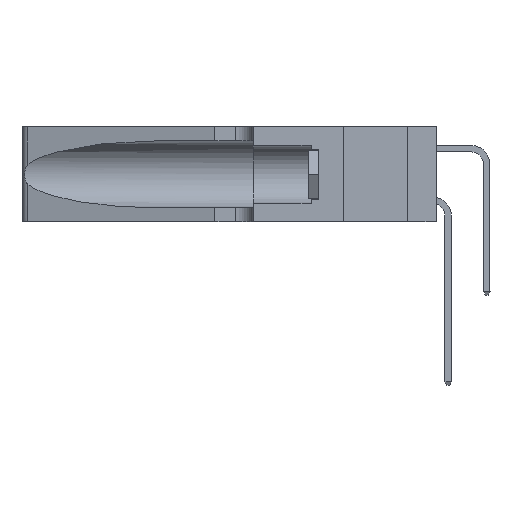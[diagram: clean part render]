
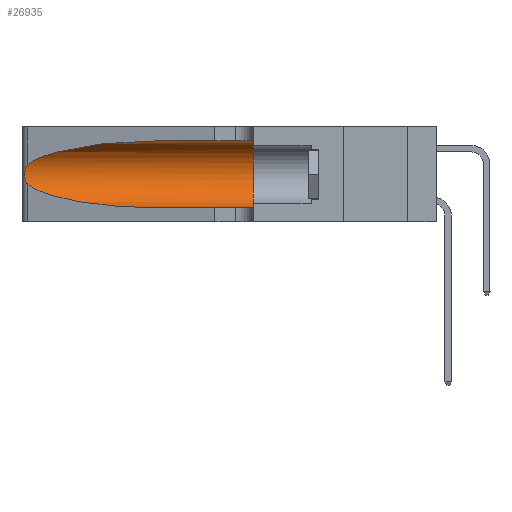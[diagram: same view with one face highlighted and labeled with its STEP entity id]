
A CAD part, left-side view. The second image highlights one B-rep face of the part: STEP entity #26935.
In plain terms, the highlighted cylindrical face has radius 3.308 mm (diameter 6.617 mm), a partial arc.
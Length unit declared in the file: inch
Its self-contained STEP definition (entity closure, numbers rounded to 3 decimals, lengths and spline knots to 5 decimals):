
#251 = ORIENTED_EDGE ( 'NONE', *, *, #4112, .T. ) ;
#1411 = CARTESIAN_POINT ( 'NONE',  ( 0.1305, 1.61858, 0.185 ) ) ;
#1829 = CARTESIAN_POINT ( 'NONE',  ( 0.25487, 1.22718, 0.14631 ) ) ;
#2220 = CARTESIAN_POINT ( 'NONE',  ( 0.25487, 1.22718, 0.14631 ) ) ;
#2361 = EDGE_CURVE ( 'NONE', #14795, #5039, #16998, .T. ) ;
#3120 = VERTEX_POINT ( 'NONE', #29177 ) ;
#3632 = CARTESIAN_POINT ( 'NONE',  ( 0.1305, 0.72297, 0.31525 ) ) ;
#4112 = EDGE_CURVE ( 'NONE', #5039, #3120, #10469, .T. ) ;
#4532 = CARTESIAN_POINT ( 'NONE',  ( 0.25639, 1.23184, 0.21858 ) ) ;
#4702 = DIRECTION ( 'NONE',  ( 0., -1., 0. ) ) ;
#5038 = EDGE_CURVE ( 'NONE', #13819, #35014, #19594, .T. ) ;
#5039 = VERTEX_POINT ( 'NONE', #11782 ) ;
#5859 = LINE ( 'NONE', #15915, #34793 ) ;
#6464 = CARTESIAN_POINT ( 'NONE',  ( 0.18966, 0.96281, 0.31525 ) ) ;
#7386 = CARTESIAN_POINT ( 'NONE',  ( 0.25854, 1.2359, 0.20912 ) ) ;
#7924 = CARTESIAN_POINT ( 'NONE',  ( 0.1305, 0.72297, 0.05475 ) ) ;
#8695 = CIRCLE ( 'NONE', #29893, 0.13025 ) ;
#9926 = DIRECTION ( 'NONE',  ( 0., 0., -1. ) ) ;
#10215 = CARTESIAN_POINT ( 'NONE',  ( 0.26075, 1.23896, 0.19203 ) ) ;
#10469 =( BOUNDED_CURVE ( )  B_SPLINE_CURVE ( 3, ( #2220, #21920, #24758, #7924 ),
 .UNSPECIFIED., .F., .F. ) 
 B_SPLINE_CURVE_WITH_KNOTS ( ( 4, 4 ),
 ( 3.44316, 4.71239 ),
 .UNSPECIFIED. ) 
 CURVE ( )  GEOMETRIC_REPRESENTATION_ITEM ( )  RATIONAL_B_SPLINE_CURVE ( ( 1., 0.87, 0.87, 1. ) ) 
 REPRESENTATION_ITEM ( '' )  );
#11574 =( BOUNDED_CURVE ( )  B_SPLINE_CURVE ( 3, ( #3632, #6464, #14979, #34494 ),
 .UNSPECIFIED., .F., .T. ) 
 B_SPLINE_CURVE_WITH_KNOTS ( ( 4, 4 ),
 ( 1.5708, 2.84003 ),
 .UNSPECIFIED. ) 
 CURVE ( )  GEOMETRIC_REPRESENTATION_ITEM ( )  RATIONAL_B_SPLINE_CURVE ( ( 1., 0.87, 0.87, 1. ) ) 
 REPRESENTATION_ITEM ( '' )  );
#11602 = DIRECTION ( 'NONE',  ( 0., 1., 0. ) ) ;
#11782 = CARTESIAN_POINT ( 'NONE',  ( 0.25487, 1.22718, 0.14631 ) ) ;
#12039 = CARTESIAN_POINT ( 'NONE',  ( 0.25487, 1.22718, 0.22369 ) ) ;
#12203 = CARTESIAN_POINT ( 'NONE',  ( 0.1305, 0.35, 0.31525 ) ) ;
#12540 = FACE_OUTER_BOUND ( 'NONE', #31478, .T. ) ;
#13046 = CARTESIAN_POINT ( 'NONE',  ( 0.26017, 1.23833, 0.17102 ) ) ;
#13693 = CARTESIAN_POINT ( 'NONE',  ( 0.1305, 0.72297, 0.31525 ) ) ;
#13819 = VERTEX_POINT ( 'NONE', #13693 ) ;
#14145 = ORIENTED_EDGE ( 'NONE', *, *, #5038, .F. ) ;
#14795 = VERTEX_POINT ( 'NONE', #12039 ) ;
#14979 = CARTESIAN_POINT ( 'NONE',  ( 0.2373, 1.15595, 0.28018 ) ) ;
#15858 = CARTESIAN_POINT ( 'NONE',  ( 0.25789, 1.23486, 0.15765 ) ) ;
#15915 = CARTESIAN_POINT ( 'NONE',  ( 0.1305, 1.61858, 0.05475 ) ) ;
#16998 = B_SPLINE_CURVE_WITH_KNOTS ( 'NONE', 3,
 ( #35282, #21401, #4532, #24237, #7386, #27033, #10215, #29806, #13046, #32613, #15858, #35395, #18716, #1829 ),
 .UNSPECIFIED., .F., .F.,
 ( 4, 2, 2, 2, 2, 2, 4 ),
 ( 0., 0.00027, 0.00053, 0.00107, 0.0016, 0.00187, 0.00214 ),
 .UNSPECIFIED. ) ;
#18716 = CARTESIAN_POINT ( 'NONE',  ( 0.25555, 1.22993, 0.14849 ) ) ;
#19594 = LINE ( 'NONE', #28569, #33545 ) ;
#19875 = ORIENTED_EDGE ( 'NONE', *, *, #2361, .T. ) ;
#21401 = CARTESIAN_POINT ( 'NONE',  ( 0.25555, 1.22994, 0.2215 ) ) ;
#21920 = CARTESIAN_POINT ( 'NONE',  ( 0.2373, 1.15595, 0.08982 ) ) ;
#22706 = ORIENTED_EDGE ( 'NONE', *, *, #25441, .F. ) ;
#24237 = CARTESIAN_POINT ( 'NONE',  ( 0.25787, 1.23484, 0.2124 ) ) ;
#24747 = VERTEX_POINT ( 'NONE', #28201 ) ;
#24758 = CARTESIAN_POINT ( 'NONE',  ( 0.18966, 0.96281, 0.05475 ) ) ;
#24858 = CYLINDRICAL_SURFACE ( 'NONE', #27260, 0.13025 ) ;
#25441 = EDGE_CURVE ( 'NONE', #35014, #24747, #8695, .T. ) ;
#26743 = DIRECTION ( 'NONE',  ( 0., -1., 0. ) ) ;
#26814 = EDGE_CURVE ( 'NONE', #13819, #14795, #11574, .T. ) ;
#26935 = ADVANCED_FACE ( 'NONE', ( #12540 ), #24858, .F. ) ;
#27033 = CARTESIAN_POINT ( 'NONE',  ( 0.26018, 1.23835, 0.19895 ) ) ;
#27260 = AXIS2_PLACEMENT_3D ( 'NONE', #1411, #26743, #9926 ) ;
#28201 = CARTESIAN_POINT ( 'NONE',  ( 0.1305, 0.35, 0.05475 ) ) ;
#28391 = CARTESIAN_POINT ( 'NONE',  ( 0.1305, 0.35, 0.185 ) ) ;
#28569 = CARTESIAN_POINT ( 'NONE',  ( 0.1305, 1.61858, 0.31525 ) ) ;
#29177 = CARTESIAN_POINT ( 'NONE',  ( 0.1305, 0.72297, 0.05475 ) ) ;
#29465 = EDGE_CURVE ( 'NONE', #3120, #24747, #5859, .T. ) ;
#29806 = CARTESIAN_POINT ( 'NONE',  ( 0.26075, 1.23896, 0.178 ) ) ;
#29893 = AXIS2_PLACEMENT_3D ( 'NONE', #28391, #11602, #31183 ) ;
#31183 = DIRECTION ( 'NONE',  ( 0., 0., 1. ) ) ;
#31236 = DIRECTION ( 'NONE',  ( 0., -1., 0. ) ) ;
#31405 = ORIENTED_EDGE ( 'NONE', *, *, #26814, .T. ) ;
#31478 = EDGE_LOOP ( 'NONE', ( #31405, #19875, #251, #31598, #22706, #14145 ) ) ;
#31598 = ORIENTED_EDGE ( 'NONE', *, *, #29465, .T. ) ;
#32613 = CARTESIAN_POINT ( 'NONE',  ( 0.25856, 1.23593, 0.16098 ) ) ;
#33545 = VECTOR ( 'NONE', #31236, 39.37008 ) ;
#34494 = CARTESIAN_POINT ( 'NONE',  ( 0.25487, 1.22718, 0.22369 ) ) ;
#34793 = VECTOR ( 'NONE', #4702, 39.37008 ) ;
#35014 = VERTEX_POINT ( 'NONE', #12203 ) ;
#35282 = CARTESIAN_POINT ( 'NONE',  ( 0.25487, 1.22718, 0.22369 ) ) ;
#35395 = CARTESIAN_POINT ( 'NONE',  ( 0.25639, 1.23186, 0.15144 ) ) ;
